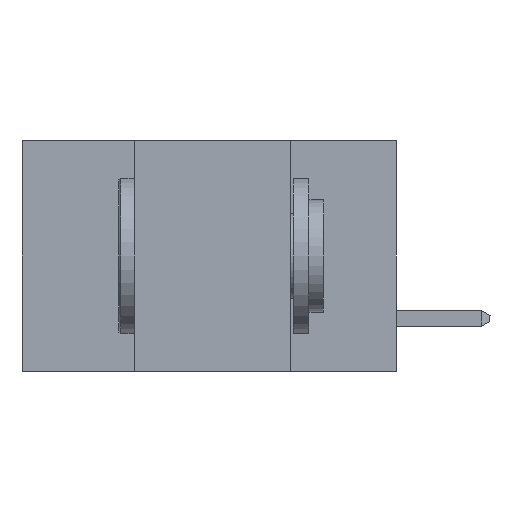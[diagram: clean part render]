
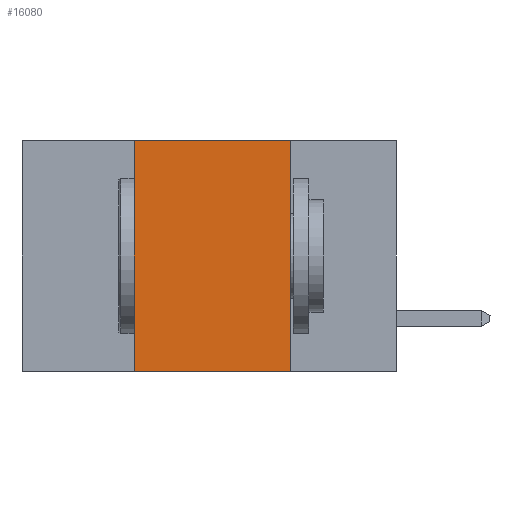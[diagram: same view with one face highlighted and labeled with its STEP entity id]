
A CAD part, left-side view. The second image highlights one B-rep face of the part: STEP entity #16080.
In plain terms, the highlighted planar face has unit normal (-1, 0, 0).
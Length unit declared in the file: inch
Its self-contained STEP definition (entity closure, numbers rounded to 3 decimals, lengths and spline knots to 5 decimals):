
#552 = DIRECTION ( 'NONE',  ( 0., 0., -1. ) ) ;
#1324 = DIRECTION ( 'NONE',  ( 0., 0., 1. ) ) ;
#2103 = CARTESIAN_POINT ( 'NONE',  ( 0., 0.17, 0. ) ) ;
#2263 = CARTESIAN_POINT ( 'NONE',  ( 0., 0.42, -0.37 ) ) ;
#2651 = VECTOR ( 'NONE', #11703, 39.37008 ) ;
#3286 = ORIENTED_EDGE ( 'NONE', *, *, #5784, .T. ) ;
#3476 = CARTESIAN_POINT ( 'NONE',  ( 0., 0.17, -0.37 ) ) ;
#3574 = ORIENTED_EDGE ( 'NONE', *, *, #10765, .F. ) ;
#4460 = CARTESIAN_POINT ( 'NONE',  ( 0., 0.6, 0. ) ) ;
#5455 = VERTEX_POINT ( 'NONE', #7289 ) ;
#5784 = EDGE_CURVE ( 'NONE', #7870, #13337, #6732, .T. ) ;
#6037 = AXIS2_PLACEMENT_3D ( 'NONE', #13712, #11957, #552 ) ;
#6732 = LINE ( 'NONE', #8152, #19624 ) ;
#7289 = CARTESIAN_POINT ( 'NONE',  ( 0., 0.42, 0. ) ) ;
#7632 = LINE ( 'NONE', #4460, #14012 ) ;
#7870 = VERTEX_POINT ( 'NONE', #2263 ) ;
#8152 = CARTESIAN_POINT ( 'NONE',  ( 0., 0.6, -0.37 ) ) ;
#9918 = DIRECTION ( 'NONE',  ( 0., -1., 0. ) ) ;
#10578 = VECTOR ( 'NONE', #1324, 39.37008 ) ;
#10765 = EDGE_CURVE ( 'NONE', #11346, #13337, #19935, .T. ) ;
#11346 = VERTEX_POINT ( 'NONE', #2103 ) ;
#11703 = DIRECTION ( 'NONE',  ( 0., 0., -1. ) ) ;
#11957 = DIRECTION ( 'NONE',  ( 1., 0., 0. ) ) ;
#12355 = ORIENTED_EDGE ( 'NONE', *, *, #15560, .F. ) ;
#12709 = CARTESIAN_POINT ( 'NONE',  ( 0., 0.17, -0.37 ) ) ;
#13337 = VERTEX_POINT ( 'NONE', #12709 ) ;
#13712 = CARTESIAN_POINT ( 'NONE',  ( 0., 0.6, 0. ) ) ;
#14012 = VECTOR ( 'NONE', #14634, 39.37008 ) ;
#14634 = DIRECTION ( 'NONE',  ( 0., -1., 0. ) ) ;
#14686 = EDGE_LOOP ( 'NONE', ( #3574, #20966, #12355, #3286 ) ) ;
#14810 = CARTESIAN_POINT ( 'NONE',  ( 0., 0.42, -0.37 ) ) ;
#15560 = EDGE_CURVE ( 'NONE', #7870, #5455, #19528, .T. ) ;
#16080 = ADVANCED_FACE ( 'NONE', ( #17217 ), #20611, .F. ) ;
#17217 = FACE_OUTER_BOUND ( 'NONE', #14686, .T. ) ;
#19528 = LINE ( 'NONE', #14810, #10578 ) ;
#19624 = VECTOR ( 'NONE', #9918, 39.37008 ) ;
#19935 = LINE ( 'NONE', #3476, #2651 ) ;
#20611 = PLANE ( 'NONE',  #6037 ) ;
#20966 = ORIENTED_EDGE ( 'NONE', *, *, #21520, .F. ) ;
#21520 = EDGE_CURVE ( 'NONE', #5455, #11346, #7632, .T. ) ;
